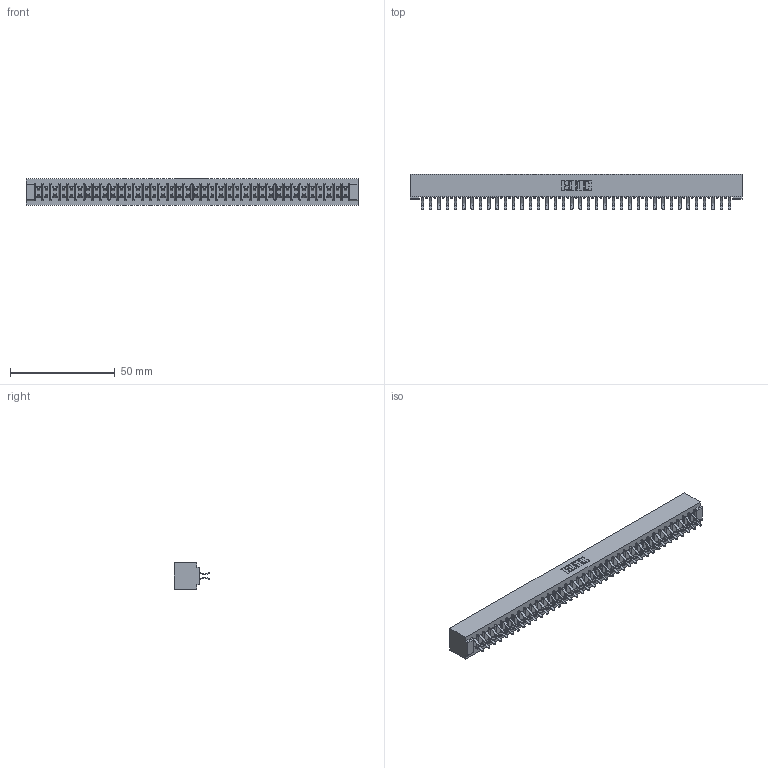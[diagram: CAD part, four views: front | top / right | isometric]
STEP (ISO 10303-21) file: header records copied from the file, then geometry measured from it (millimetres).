
FILE_DESCRIPTION (( 'STEP AP203' ), '1' );
FILE_NAME ('357-076-456-201.STEP', '2020-10-04T15:15:26', ( '' ), ( '' ), 'SwSTEP 2.0', 'SolidWorks 2020', '' );
FILE_SCHEMA (( 'CONFIG_CONTROL_DESIGN' ));
Length unit declared in the file: inch
Products named in the file (3): 307 Part_No Mounting Lugs; 357-076-456-201; 307-290-001_556
Assembly tree (77 placements, depth 2):
  357-076-456-201
    307 Part_No Mounting Lugs
    307-290-001_556  x76
Bounding box: 158.45 x 16.97 x 12.7 mm (x, y, z)
Volume: 17354.2 mm3; surface area: 21267.8 mm2
Topology: 77 solids, 77 shells, 3949 faces, 11091 edges, 7186 vertices
Faces by surface type: plane 2574, cylinder 1297, sphere 78
Entity records: 34112 total; most frequent: CARTESIAN_POINT 5578, ORIENTED_EDGE 5526, DIRECTION 5465, EDGE_CURVE 2763, LINE 2119, VECTOR 2119, VERTEX_POINT 1786, AXIS2_PLACEMENT_3D 1673
